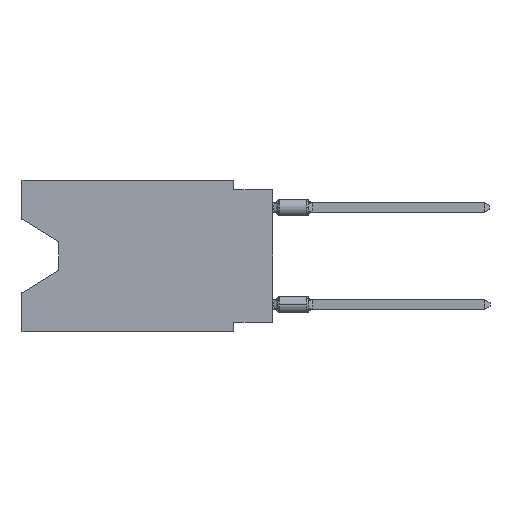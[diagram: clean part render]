
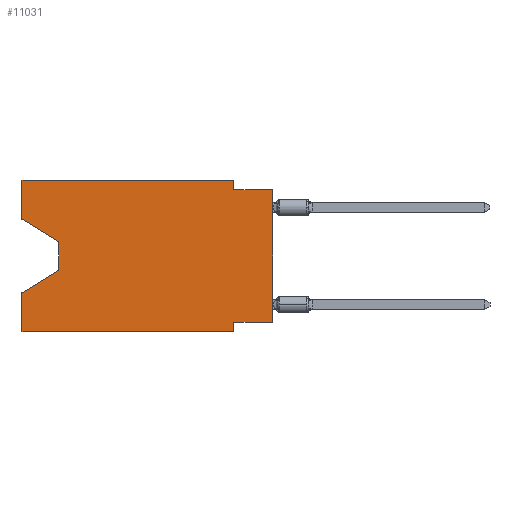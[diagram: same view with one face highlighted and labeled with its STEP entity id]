
A CAD part, left-side view. The second image highlights one B-rep face of the part: STEP entity #11031.
In plain terms, the highlighted planar face has unit normal (-1, 0, 0).
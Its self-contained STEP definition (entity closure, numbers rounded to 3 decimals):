
#139 = VECTOR ( 'NONE', #4916, 1000. ) ;
#261 = VERTEX_POINT ( 'NONE', #6843 ) ;
#262 = ORIENTED_EDGE ( 'NONE', *, *, #10548, .F. ) ;
#611 = AXIS2_PLACEMENT_3D ( 'NONE', #16088, #6799, #12315 ) ;
#765 = VERTEX_POINT ( 'NONE', #3845 ) ;
#979 = VECTOR ( 'NONE', #20248, 1000. ) ;
#1120 = ORIENTED_EDGE ( 'NONE', *, *, #3561, .F. ) ;
#1746 = CARTESIAN_POINT ( 'NONE',  ( 0., 0., 0. ) ) ;
#1784 = EDGE_CURVE ( 'NONE', #5644, #5669, #12178, .T. ) ;
#1789 = LINE ( 'NONE', #20177, #16576 ) ;
#2554 = LINE ( 'NONE', #15508, #2942 ) ;
#2556 = LINE ( 'NONE', #4513, #13445 ) ;
#2739 = CARTESIAN_POINT ( 'NONE',  ( 0., 16.383, -9.906 ) ) ;
#2881 = CARTESIAN_POINT ( 'NONE',  ( 0., 0., -0.635 ) ) ;
#2942 = VECTOR ( 'NONE', #23481, 1000. ) ;
#3488 = PLANE ( 'NONE',  #611 ) ;
#3561 = EDGE_CURVE ( 'NONE', #10148, #18335, #14696, .T. ) ;
#3617 = VECTOR ( 'NONE', #5372, 1000. ) ;
#3845 = CARTESIAN_POINT ( 'NONE',  ( 0., 16.383, 0. ) ) ;
#4308 = EDGE_CURVE ( 'NONE', #18367, #20299, #19925, .T. ) ;
#4513 = CARTESIAN_POINT ( 'NONE',  ( 0., 16.383, -9.906 ) ) ;
#4861 = LINE ( 'NONE', #8409, #23986 ) ;
#4916 = DIRECTION ( 'NONE',  ( 0., 0., -1. ) ) ;
#5372 = DIRECTION ( 'NONE',  ( 0., 0.855, -0.519 ) ) ;
#5408 = CARTESIAN_POINT ( 'NONE',  ( 0., 13.97, -5.893 ) ) ;
#5478 = ORIENTED_EDGE ( 'NONE', *, *, #21780, .T. ) ;
#5612 = VECTOR ( 'NONE', #12545, 1000. ) ;
#5644 = VERTEX_POINT ( 'NONE', #16715 ) ;
#5669 = VERTEX_POINT ( 'NONE', #15213 ) ;
#5708 = ORIENTED_EDGE ( 'NONE', *, *, #18600, .T. ) ;
#6166 = VERTEX_POINT ( 'NONE', #9577 ) ;
#6396 = ORIENTED_EDGE ( 'NONE', *, *, #10438, .T. ) ;
#6799 = DIRECTION ( 'NONE',  ( 1., 0., 0. ) ) ;
#6843 = CARTESIAN_POINT ( 'NONE',  ( 0., 2.54, -9.906 ) ) ;
#7044 = VECTOR ( 'NONE', #23567, 1000. ) ;
#7132 = EDGE_CURVE ( 'NONE', #20299, #18089, #23191, .T. ) ;
#7850 = CARTESIAN_POINT ( 'NONE',  ( 0., 2.54, 0. ) ) ;
#7852 = ORIENTED_EDGE ( 'NONE', *, *, #1784, .T. ) ;
#8409 = CARTESIAN_POINT ( 'NONE',  ( 0., 2.54, -9.906 ) ) ;
#8754 = FACE_OUTER_BOUND ( 'NONE', #22730, .T. ) ;
#8824 = LINE ( 'NONE', #21804, #139 ) ;
#9087 = LINE ( 'NONE', #1746, #979 ) ;
#9092 = CARTESIAN_POINT ( 'NONE',  ( 0., 2.54, -0.635 ) ) ;
#9577 = CARTESIAN_POINT ( 'NONE',  ( 0., 0., -9.271 ) ) ;
#10148 = VERTEX_POINT ( 'NONE', #2739 ) ;
#10438 = EDGE_CURVE ( 'NONE', #6166, #18089, #9087, .T. ) ;
#10548 = EDGE_CURVE ( 'NONE', #765, #18367, #2554, .T. ) ;
#10615 = CARTESIAN_POINT ( 'NONE',  ( 0., 2.54, 0. ) ) ;
#11017 = ORIENTED_EDGE ( 'NONE', *, *, #16238, .F. ) ;
#11031 = ADVANCED_FACE ( 'NONE', ( #8754 ), #3488, .F. ) ;
#11049 = CARTESIAN_POINT ( 'NONE',  ( 0., 16.383, 0. ) ) ;
#12178 = LINE ( 'NONE', #21848, #5612 ) ;
#12315 = DIRECTION ( 'NONE',  ( 0., 0., -1. ) ) ;
#12545 = DIRECTION ( 'NONE',  ( 0., -0.855, -0.519 ) ) ;
#12966 = LINE ( 'NONE', #18370, #3617 ) ;
#13218 = VECTOR ( 'NONE', #17452, 1000. ) ;
#13445 = VECTOR ( 'NONE', #17252, 1000. ) ;
#13752 = CARTESIAN_POINT ( 'NONE',  ( 0., 2.54, -9.271 ) ) ;
#13755 = DIRECTION ( 'NONE',  ( 0., -1., 0. ) ) ;
#13761 = EDGE_CURVE ( 'NONE', #6166, #16612, #21123, .T. ) ;
#13908 = ORIENTED_EDGE ( 'NONE', *, *, #23790, .T. ) ;
#13912 = DIRECTION ( 'NONE',  ( 0., 0., -1. ) ) ;
#14625 = DIRECTION ( 'NONE',  ( 0., 0., 1. ) ) ;
#14696 = LINE ( 'NONE', #11049, #7044 ) ;
#14702 = VECTOR ( 'NONE', #18080, 1000. ) ;
#14918 = CARTESIAN_POINT ( 'NONE',  ( 0., 16.383, -7.36 ) ) ;
#15213 = CARTESIAN_POINT ( 'NONE',  ( 0., 13.97, -4.013 ) ) ;
#15508 = CARTESIAN_POINT ( 'NONE',  ( 0., 16.383, 0. ) ) ;
#16088 = CARTESIAN_POINT ( 'NONE',  ( 0., 16.383, 0. ) ) ;
#16238 = EDGE_CURVE ( 'NONE', #16612, #261, #4861, .T. ) ;
#16385 = EDGE_CURVE ( 'NONE', #5644, #765, #1789, .T. ) ;
#16576 = VECTOR ( 'NONE', #14625, 1000. ) ;
#16612 = VERTEX_POINT ( 'NONE', #13752 ) ;
#16715 = CARTESIAN_POINT ( 'NONE',  ( 0., 16.383, -2.546 ) ) ;
#17252 = DIRECTION ( 'NONE',  ( 0., -1., 0. ) ) ;
#17452 = DIRECTION ( 'NONE',  ( 0., 1., 0. ) ) ;
#18080 = DIRECTION ( 'NONE',  ( 0., 0., -1. ) ) ;
#18089 = VERTEX_POINT ( 'NONE', #23658 ) ;
#18335 = VERTEX_POINT ( 'NONE', #14918 ) ;
#18367 = VERTEX_POINT ( 'NONE', #7850 ) ;
#18370 = CARTESIAN_POINT ( 'NONE',  ( 0., 13.97, -5.893 ) ) ;
#18564 = ORIENTED_EDGE ( 'NONE', *, *, #13761, .F. ) ;
#18600 = EDGE_CURVE ( 'NONE', #23108, #18335, #12966, .T. ) ;
#18895 = ORIENTED_EDGE ( 'NONE', *, *, #4308, .F. ) ;
#18896 = ORIENTED_EDGE ( 'NONE', *, *, #7132, .F. ) ;
#19925 = LINE ( 'NONE', #10615, #14702 ) ;
#20177 = CARTESIAN_POINT ( 'NONE',  ( 0., 16.383, 0. ) ) ;
#20248 = DIRECTION ( 'NONE',  ( 0., 0., 1. ) ) ;
#20299 = VERTEX_POINT ( 'NONE', #9092 ) ;
#21123 = LINE ( 'NONE', #21243, #13218 ) ;
#21243 = CARTESIAN_POINT ( 'NONE',  ( 0., 0., -9.271 ) ) ;
#21780 = EDGE_CURVE ( 'NONE', #5669, #23108, #8824, .T. ) ;
#21804 = CARTESIAN_POINT ( 'NONE',  ( 0., 13.97, -4.013 ) ) ;
#21848 = CARTESIAN_POINT ( 'NONE',  ( 0., 16.383, -2.546 ) ) ;
#22637 = VECTOR ( 'NONE', #13755, 1000. ) ;
#22730 = EDGE_LOOP ( 'NONE', ( #7852, #5478, #5708, #1120, #13908, #11017, #18564, #6396, #18896, #18895, #262, #23235 ) ) ;
#23108 = VERTEX_POINT ( 'NONE', #5408 ) ;
#23191 = LINE ( 'NONE', #2881, #22637 ) ;
#23235 = ORIENTED_EDGE ( 'NONE', *, *, #16385, .F. ) ;
#23481 = DIRECTION ( 'NONE',  ( 0., -1., 0. ) ) ;
#23567 = DIRECTION ( 'NONE',  ( 0., 0., 1. ) ) ;
#23658 = CARTESIAN_POINT ( 'NONE',  ( 0., 0., -0.635 ) ) ;
#23790 = EDGE_CURVE ( 'NONE', #10148, #261, #2556, .T. ) ;
#23986 = VECTOR ( 'NONE', #13912, 1000. ) ;
